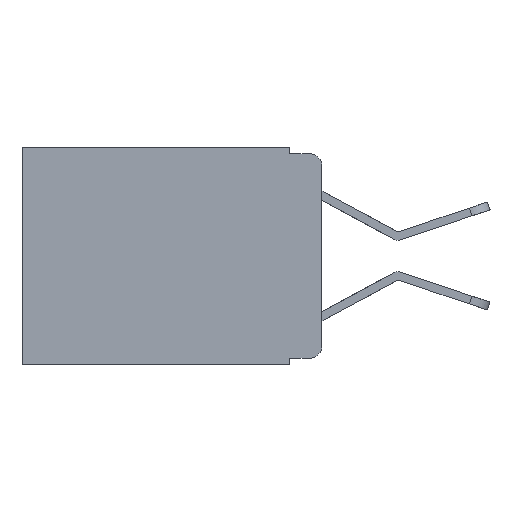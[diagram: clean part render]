
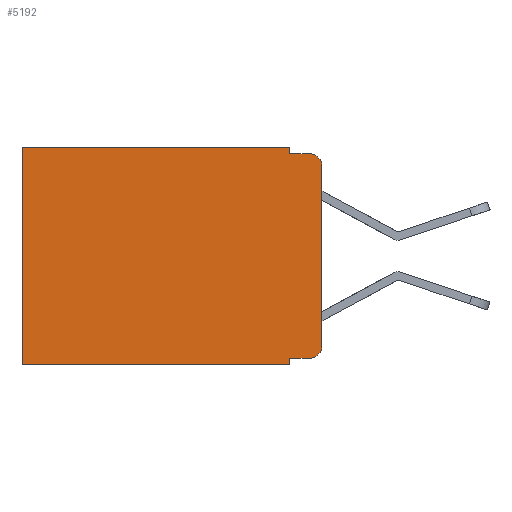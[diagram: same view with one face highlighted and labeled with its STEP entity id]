
A CAD part, left-side view. The second image highlights one B-rep face of the part: STEP entity #5192.
In plain terms, the highlighted planar face has unit normal (-1, 0, 0).
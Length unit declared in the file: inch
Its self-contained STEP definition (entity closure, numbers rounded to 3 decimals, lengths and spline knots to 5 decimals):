
#38 = DIRECTION ( 'NONE',  ( -1., 0., 0. ) ) ;
#41 = VECTOR ( 'NONE', #4813, 39.37008 ) ;
#82 = CARTESIAN_POINT ( 'NONE',  ( 0.298, 0., -0.343 ) ) ;
#95 = ORIENTED_EDGE ( 'NONE', *, *, #5392, .F. ) ;
#150 = CARTESIAN_POINT ( 'NONE',  ( 0.298, 0.02, -0.333 ) ) ;
#226 = VECTOR ( 'NONE', #7719, 39.37008 ) ;
#234 = FACE_OUTER_BOUND ( 'NONE', #4768, .T. ) ;
#281 = EDGE_CURVE ( 'NONE', #7383, #11256, #2521, .T. ) ;
#301 = DIRECTION ( 'NONE',  ( 1., 0., 0. ) ) ;
#923 = LINE ( 'NONE', #82, #5074 ) ;
#1291 = CARTESIAN_POINT ( 'NONE',  ( 0.298, 0.473, 0. ) ) ;
#1311 = VERTEX_POINT ( 'NONE', #7777 ) ;
#1531 = DIRECTION ( 'NONE',  ( 0., 0., -1. ) ) ;
#2090 = CARTESIAN_POINT ( 'NONE',  ( 0.298, 0.051, -0.01 ) ) ;
#2118 = PLANE ( 'NONE',  #9487 ) ;
#2288 = VECTOR ( 'NONE', #8586, 39.37008 ) ;
#2445 = CARTESIAN_POINT ( 'NONE',  ( 0.298, 0., 0. ) ) ;
#2521 = LINE ( 'NONE', #3339, #226 ) ;
#2608 = VECTOR ( 'NONE', #1531, 39.37008 ) ;
#2872 = EDGE_CURVE ( 'NONE', #3328, #1311, #5775, .T. ) ;
#3054 = DIRECTION ( 'NONE',  ( 0., 0., -1. ) ) ;
#3238 = CIRCLE ( 'NONE', #10683, 0.02 ) ;
#3328 = VERTEX_POINT ( 'NONE', #4788 ) ;
#3339 = CARTESIAN_POINT ( 'NONE',  ( 0.298, 0., 0. ) ) ;
#3371 = VECTOR ( 'NONE', #6023, 39.37008 ) ;
#3461 = LINE ( 'NONE', #5041, #2288 ) ;
#3656 = EDGE_CURVE ( 'NONE', #5667, #5640, #11071, .T. ) ;
#3658 = DIRECTION ( 'NONE',  ( 0., 1., 0. ) ) ;
#3857 = CARTESIAN_POINT ( 'NONE',  ( 0.298, 0.051, -0.333 ) ) ;
#4160 = CARTESIAN_POINT ( 'NONE',  ( 0.298, 0.051, 0. ) ) ;
#4285 = CARTESIAN_POINT ( 'NONE',  ( 0.298, 0.02, -0.313 ) ) ;
#4412 = EDGE_CURVE ( 'NONE', #5640, #5619, #6707, .T. ) ;
#4768 = EDGE_LOOP ( 'NONE', ( #95, #5741, #9083, #9024, #6880, #5042, #6381, #7391, #7369, #5410 ) ) ;
#4788 = CARTESIAN_POINT ( 'NONE',  ( 0.298, 0.051, -0.01 ) ) ;
#4813 = DIRECTION ( 'NONE',  ( 0., 0., -1. ) ) ;
#4903 = EDGE_CURVE ( 'NONE', #5667, #10085, #9509, .T. ) ;
#4965 = DIRECTION ( 'NONE',  ( 0., -1., 0. ) ) ;
#4981 = VERTEX_POINT ( 'NONE', #7667 ) ;
#5041 = CARTESIAN_POINT ( 'NONE',  ( 0.298, 0.051, 0. ) ) ;
#5042 = ORIENTED_EDGE ( 'NONE', *, *, #10666, .T. ) ;
#5074 = VECTOR ( 'NONE', #3658, 39.37008 ) ;
#5192 = ADVANCED_FACE ( 'NONE', ( #234 ), #2118, .F. ) ;
#5392 = EDGE_CURVE ( 'NONE', #10210, #5619, #10436, .T. ) ;
#5410 = ORIENTED_EDGE ( 'NONE', *, *, #4412, .T. ) ;
#5619 = VERTEX_POINT ( 'NONE', #6539 ) ;
#5640 = VERTEX_POINT ( 'NONE', #150 ) ;
#5667 = VERTEX_POINT ( 'NONE', #3857 ) ;
#5684 = CARTESIAN_POINT ( 'NONE',  ( 0.298, 0., 0. ) ) ;
#5741 = ORIENTED_EDGE ( 'NONE', *, *, #10943, .T. ) ;
#5775 = LINE ( 'NONE', #2090, #9383 ) ;
#6023 = DIRECTION ( 'NONE',  ( 0., 0., -1. ) ) ;
#6225 = VECTOR ( 'NONE', #7339, 39.37008 ) ;
#6381 = ORIENTED_EDGE ( 'NONE', *, *, #8414, .F. ) ;
#6539 = CARTESIAN_POINT ( 'NONE',  ( 0.298, 0., -0.313 ) ) ;
#6639 = CARTESIAN_POINT ( 'NONE',  ( 0.298, 0.051, -0.333 ) ) ;
#6707 = CIRCLE ( 'NONE', #8738, 0.02 ) ;
#6880 = ORIENTED_EDGE ( 'NONE', *, *, #281, .T. ) ;
#7063 = CARTESIAN_POINT ( 'NONE',  ( 0.298, 0.02, -0.03 ) ) ;
#7339 = DIRECTION ( 'NONE',  ( 0., -1., 0. ) ) ;
#7369 = ORIENTED_EDGE ( 'NONE', *, *, #3656, .T. ) ;
#7383 = VERTEX_POINT ( 'NONE', #8376 ) ;
#7391 = ORIENTED_EDGE ( 'NONE', *, *, #4903, .F. ) ;
#7667 = CARTESIAN_POINT ( 'NONE',  ( 0.298, 0.473, -0.343 ) ) ;
#7719 = DIRECTION ( 'NONE',  ( 0., 1., 0. ) ) ;
#7777 = CARTESIAN_POINT ( 'NONE',  ( 0.298, 0.02, -0.01 ) ) ;
#7848 = DIRECTION ( 'NONE',  ( 0., 0., -1. ) ) ;
#7990 = DIRECTION ( 'NONE',  ( 0., 0., -1. ) ) ;
#8376 = CARTESIAN_POINT ( 'NONE',  ( 0.298, 0.051, 0. ) ) ;
#8414 = EDGE_CURVE ( 'NONE', #10085, #4981, #923, .T. ) ;
#8586 = DIRECTION ( 'NONE',  ( 0., 0., -1. ) ) ;
#8738 = AXIS2_PLACEMENT_3D ( 'NONE', #4285, #9636, #7848 ) ;
#9024 = ORIENTED_EDGE ( 'NONE', *, *, #10482, .F. ) ;
#9083 = ORIENTED_EDGE ( 'NONE', *, *, #2872, .F. ) ;
#9114 = CARTESIAN_POINT ( 'NONE',  ( 0.298, 0., -0.03 ) ) ;
#9163 = LINE ( 'NONE', #1291, #41 ) ;
#9383 = VECTOR ( 'NONE', #4965, 39.37008 ) ;
#9487 = AXIS2_PLACEMENT_3D ( 'NONE', #5684, #301, #3054 ) ;
#9509 = LINE ( 'NONE', #4160, #2608 ) ;
#9636 = DIRECTION ( 'NONE',  ( -1., 0., 0. ) ) ;
#9869 = CARTESIAN_POINT ( 'NONE',  ( 0.298, 0.051, -0.343 ) ) ;
#10085 = VERTEX_POINT ( 'NONE', #9869 ) ;
#10210 = VERTEX_POINT ( 'NONE', #9114 ) ;
#10369 = CARTESIAN_POINT ( 'NONE',  ( 0.298, 0.473, 0. ) ) ;
#10436 = LINE ( 'NONE', #2445, #3371 ) ;
#10482 = EDGE_CURVE ( 'NONE', #7383, #3328, #3461, .T. ) ;
#10666 = EDGE_CURVE ( 'NONE', #11256, #4981, #9163, .T. ) ;
#10683 = AXIS2_PLACEMENT_3D ( 'NONE', #7063, #38, #7990 ) ;
#10943 = EDGE_CURVE ( 'NONE', #10210, #1311, #3238, .T. ) ;
#11071 = LINE ( 'NONE', #6639, #6225 ) ;
#11256 = VERTEX_POINT ( 'NONE', #10369 ) ;
